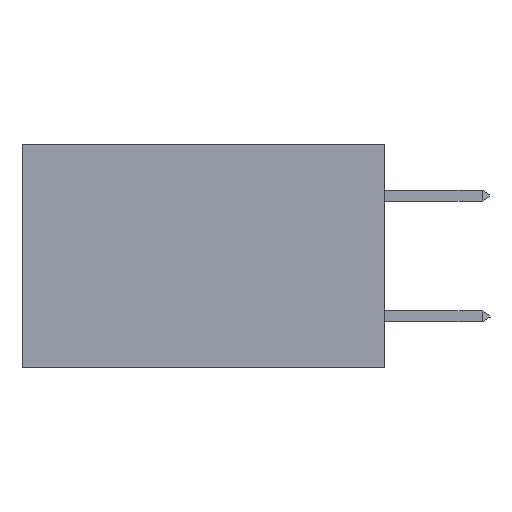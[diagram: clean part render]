
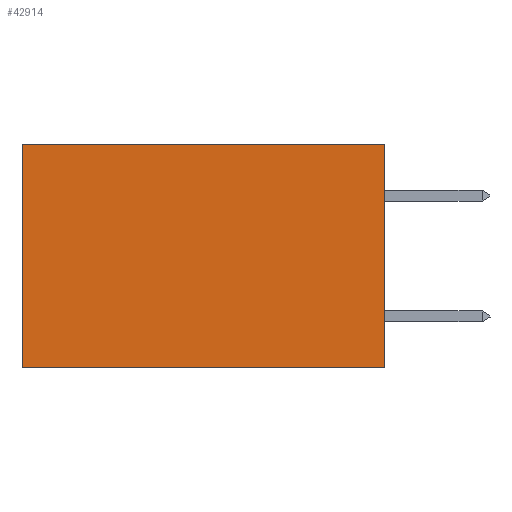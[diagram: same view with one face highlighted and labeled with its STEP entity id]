
A CAD part, left-side view. The second image highlights one B-rep face of the part: STEP entity #42914.
In plain terms, the highlighted planar face has unit normal (-1, 0, 0).
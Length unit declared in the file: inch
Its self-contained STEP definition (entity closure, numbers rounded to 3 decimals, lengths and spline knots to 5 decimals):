
#839 = CARTESIAN_POINT ( 'NONE',  ( 0.2875, 0.6, 0. ) ) ;
#1394 = EDGE_CURVE ( 'NONE', #27985, #18290, #42776, .T. ) ;
#1555 = LINE ( 'NONE', #35695, #32391 ) ;
#1719 = CARTESIAN_POINT ( 'NONE',  ( 0.2875, 0., 0. ) ) ;
#2040 = VECTOR ( 'NONE', #33970, 39.37008 ) ;
#3344 = VERTEX_POINT ( 'NONE', #34064 ) ;
#5147 = EDGE_LOOP ( 'NONE', ( #36626, #39646, #39899, #22977 ) ) ;
#5602 = CARTESIAN_POINT ( 'NONE',  ( 0.2875, 0.6, -0.37 ) ) ;
#6673 = VERTEX_POINT ( 'NONE', #36332 ) ;
#9420 = EDGE_CURVE ( 'NONE', #3344, #6673, #30673, .T. ) ;
#12451 = CARTESIAN_POINT ( 'NONE',  ( 0.2875, 0., -0.37 ) ) ;
#12759 = CARTESIAN_POINT ( 'NONE',  ( 0.2875, 0., 0. ) ) ;
#15693 = DIRECTION ( 'NONE',  ( 0., 1., 0. ) ) ;
#18290 = VERTEX_POINT ( 'NONE', #5602 ) ;
#18306 = CARTESIAN_POINT ( 'NONE',  ( 0.2875, 0.6, 0. ) ) ;
#18954 = FACE_OUTER_BOUND ( 'NONE', #5147, .T. ) ;
#21713 = DIRECTION ( 'NONE',  ( 1., 0., 0. ) ) ;
#21788 = VECTOR ( 'NONE', #32313, 39.37008 ) ;
#22977 = ORIENTED_EDGE ( 'NONE', *, *, #25356, .T. ) ;
#23076 = VECTOR ( 'NONE', #39006, 39.37008 ) ;
#25356 = EDGE_CURVE ( 'NONE', #3344, #27985, #1555, .T. ) ;
#25523 = PLANE ( 'NONE',  #25884 ) ;
#25884 = AXIS2_PLACEMENT_3D ( 'NONE', #1719, #21713, #42116 ) ;
#27985 = VERTEX_POINT ( 'NONE', #18306 ) ;
#30673 = LINE ( 'NONE', #12759, #21788 ) ;
#31946 = LINE ( 'NONE', #12451, #23076 ) ;
#32313 = DIRECTION ( 'NONE',  ( 0., 0., -1. ) ) ;
#32391 = VECTOR ( 'NONE', #15693, 39.37008 ) ;
#32865 = EDGE_CURVE ( 'NONE', #6673, #18290, #31946, .T. ) ;
#33970 = DIRECTION ( 'NONE',  ( 0., 0., -1. ) ) ;
#34064 = CARTESIAN_POINT ( 'NONE',  ( 0.2875, 0., 0. ) ) ;
#35695 = CARTESIAN_POINT ( 'NONE',  ( 0.2875, 0., 0. ) ) ;
#36332 = CARTESIAN_POINT ( 'NONE',  ( 0.2875, 0., -0.37 ) ) ;
#36626 = ORIENTED_EDGE ( 'NONE', *, *, #1394, .T. ) ;
#39006 = DIRECTION ( 'NONE',  ( 0., 1., 0. ) ) ;
#39646 = ORIENTED_EDGE ( 'NONE', *, *, #32865, .F. ) ;
#39899 = ORIENTED_EDGE ( 'NONE', *, *, #9420, .F. ) ;
#42116 = DIRECTION ( 'NONE',  ( 0., 0., -1. ) ) ;
#42776 = LINE ( 'NONE', #839, #2040 ) ;
#42914 = ADVANCED_FACE ( 'NONE', ( #18954 ), #25523, .F. ) ;
